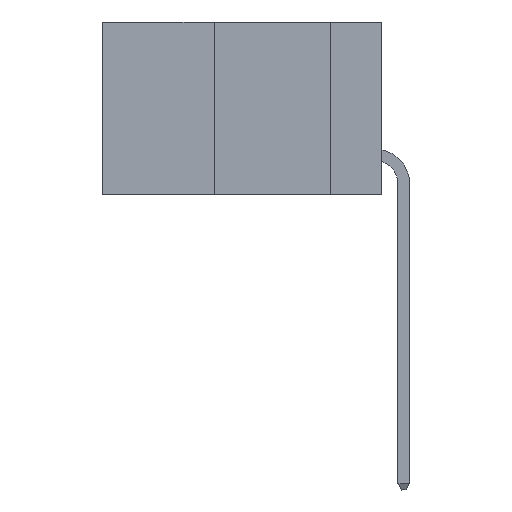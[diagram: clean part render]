
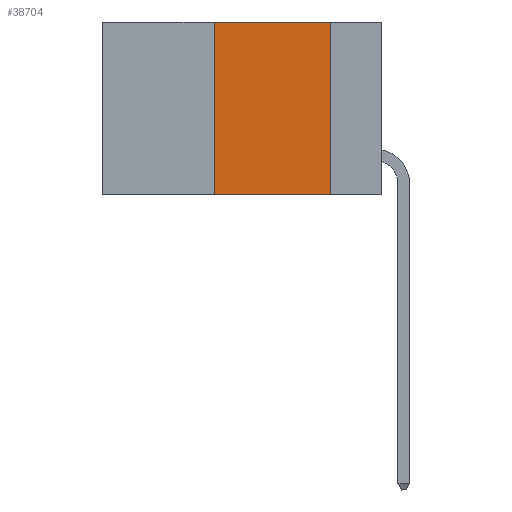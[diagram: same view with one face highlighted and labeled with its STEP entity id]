
A CAD part, left-side view. The second image highlights one B-rep face of the part: STEP entity #38704.
In plain terms, the highlighted planar face has unit normal (-1, 0, 0).
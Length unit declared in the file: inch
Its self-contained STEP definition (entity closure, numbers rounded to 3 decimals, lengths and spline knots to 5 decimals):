
#563 = VERTEX_POINT ( 'NONE', #40428 ) ;
#2398 = DIRECTION ( 'NONE',  ( 0., -1., 0. ) ) ;
#4077 = LINE ( 'NONE', #30364, #11881 ) ;
#4583 = PLANE ( 'NONE',  #5414 ) ;
#5162 = EDGE_CURVE ( 'NONE', #563, #17924, #29135, .T. ) ;
#5321 = ORIENTED_EDGE ( 'NONE', *, *, #44571, .F. ) ;
#5414 = AXIS2_PLACEMENT_3D ( 'NONE', #41214, #22789, #11770 ) ;
#5671 = ORIENTED_EDGE ( 'NONE', *, *, #5162, .T. ) ;
#6061 = LINE ( 'NONE', #22906, #26270 ) ;
#7939 = EDGE_CURVE ( 'NONE', #563, #41487, #6061, .T. ) ;
#9094 = CARTESIAN_POINT ( 'NONE',  ( 0., 0.11, 0. ) ) ;
#11770 = DIRECTION ( 'NONE',  ( 0., 0., -1. ) ) ;
#11881 = VECTOR ( 'NONE', #2398, 39.37008 ) ;
#11955 = DIRECTION ( 'NONE',  ( 0., -1., 0. ) ) ;
#14514 = VECTOR ( 'NONE', #11955, 39.37008 ) ;
#15637 = VERTEX_POINT ( 'NONE', #32174 ) ;
#17924 = VERTEX_POINT ( 'NONE', #43998 ) ;
#19456 = DIRECTION ( 'NONE',  ( 0., 0., 1. ) ) ;
#19640 = EDGE_CURVE ( 'NONE', #41487, #15637, #4077, .T. ) ;
#21139 = FACE_OUTER_BOUND ( 'NONE', #28395, .T. ) ;
#22789 = DIRECTION ( 'NONE',  ( 1., 0., 0. ) ) ;
#22906 = CARTESIAN_POINT ( 'NONE',  ( 0., 0.36, 0. ) ) ;
#24864 = CARTESIAN_POINT ( 'NONE',  ( 0., 0.36, 0. ) ) ;
#26270 = VECTOR ( 'NONE', #19456, 39.37008 ) ;
#26277 = CARTESIAN_POINT ( 'NONE',  ( 0., 0.6, -0.37 ) ) ;
#27804 = LINE ( 'NONE', #9094, #41929 ) ;
#28395 = EDGE_LOOP ( 'NONE', ( #5321, #31628, #34282, #5671 ) ) ;
#29135 = LINE ( 'NONE', #26277, #14514 ) ;
#30364 = CARTESIAN_POINT ( 'NONE',  ( 0., 0.6, 0. ) ) ;
#31628 = ORIENTED_EDGE ( 'NONE', *, *, #19640, .F. ) ;
#32174 = CARTESIAN_POINT ( 'NONE',  ( 0., 0.11, 0. ) ) ;
#34258 = DIRECTION ( 'NONE',  ( 0., 0., -1. ) ) ;
#34282 = ORIENTED_EDGE ( 'NONE', *, *, #7939, .F. ) ;
#38704 = ADVANCED_FACE ( 'NONE', ( #21139 ), #4583, .F. ) ;
#40428 = CARTESIAN_POINT ( 'NONE',  ( 0., 0.36, -0.37 ) ) ;
#41214 = CARTESIAN_POINT ( 'NONE',  ( 0., 0.6, 0. ) ) ;
#41487 = VERTEX_POINT ( 'NONE', #24864 ) ;
#41929 = VECTOR ( 'NONE', #34258, 39.37008 ) ;
#43998 = CARTESIAN_POINT ( 'NONE',  ( 0., 0.11, -0.37 ) ) ;
#44571 = EDGE_CURVE ( 'NONE', #15637, #17924, #27804, .T. ) ;
